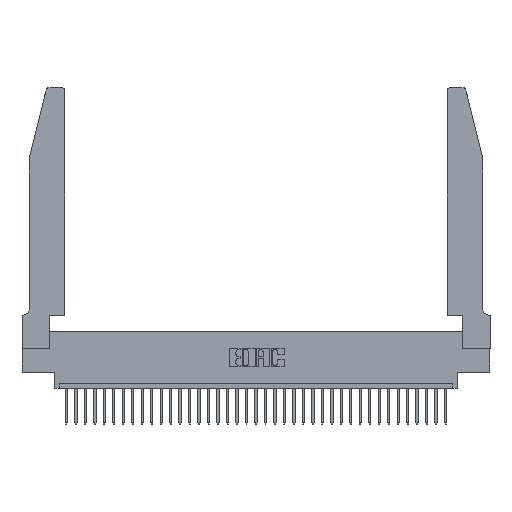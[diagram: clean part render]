
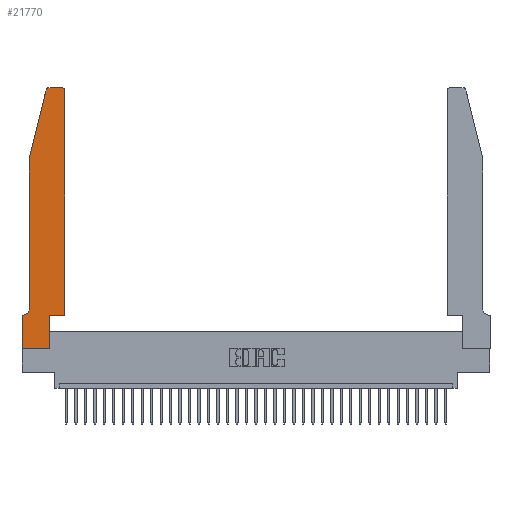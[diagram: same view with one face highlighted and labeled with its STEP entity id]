
A CAD part, top view. The second image highlights one B-rep face of the part: STEP entity #21770.
In plain terms, the highlighted planar face has unit normal (0, 0, 1).
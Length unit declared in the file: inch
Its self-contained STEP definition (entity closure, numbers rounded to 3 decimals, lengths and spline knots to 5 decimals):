
#656 = CARTESIAN_POINT ( 'NONE',  ( 0.4505, 0.35, 0.37 ) ) ;
#901 = CARTESIAN_POINT ( 'NONE',  ( 0., 0.35, 0.37 ) ) ;
#1197 = AXIS2_PLACEMENT_3D ( 'NONE', #6279, #25697, #6042 ) ;
#2085 = CARTESIAN_POINT ( 'NONE',  ( 0.0755, 0.35, 0.37 ) ) ;
#2433 = CARTESIAN_POINT ( 'NONE',  ( 0.4505, 0.35, 0.37 ) ) ;
#2552 = CARTESIAN_POINT ( 'NONE',  ( 0.4505, 0.35, 0.37 ) ) ;
#3218 = AXIS2_PLACEMENT_3D ( 'NONE', #8795, #33300, #3228 ) ;
#3228 = DIRECTION ( 'NONE',  ( 1., 0., 0. ) ) ;
#3266 = ORIENTED_EDGE ( 'NONE', *, *, #34388, .T. ) ;
#3433 = VERTEX_POINT ( 'NONE', #11619 ) ;
#3862 = DIRECTION ( 'NONE',  ( 0., -1., 0. ) ) ;
#3892 = VERTEX_POINT ( 'NONE', #28215 ) ;
#4036 = CARTESIAN_POINT ( 'NONE',  ( 0.0755, 2., 0.37 ) ) ;
#4146 = DIRECTION ( 'NONE',  ( -0.239, -0.971, 0. ) ) ;
#4921 = EDGE_CURVE ( 'NONE', #29122, #13844, #13329, .T. ) ;
#4965 = ORIENTED_EDGE ( 'NONE', *, *, #17243, .T. ) ;
#5067 = EDGE_CURVE ( 'NONE', #3433, #7374, #6825, .T. ) ;
#5284 = ORIENTED_EDGE ( 'NONE', *, *, #26502, .T. ) ;
#5329 = ORIENTED_EDGE ( 'NONE', *, *, #19090, .T. ) ;
#6042 = DIRECTION ( 'NONE',  ( 1., 0., 0. ) ) ;
#6279 = CARTESIAN_POINT ( 'NONE',  ( 0.284, 2.72, 0.37 ) ) ;
#6324 = LINE ( 'NONE', #17989, #27552 ) ;
#6640 = LINE ( 'NONE', #656, #7516 ) ;
#6825 = LINE ( 'NONE', #25083, #35454 ) ;
#7374 = VERTEX_POINT ( 'NONE', #9486 ) ;
#7516 = VECTOR ( 'NONE', #14567, 39.37008 ) ;
#7779 = AXIS2_PLACEMENT_3D ( 'NONE', #9310, #20722, #12105 ) ;
#8002 = DIRECTION ( 'NONE',  ( 1., 0., 0. ) ) ;
#8446 = DIRECTION ( 'NONE',  ( 0., 1., 0. ) ) ;
#8474 = ORIENTED_EDGE ( 'NONE', *, *, #24300, .T. ) ;
#8795 = CARTESIAN_POINT ( 'NONE',  ( 0.4205, 2.72, 0.37 ) ) ;
#9310 = CARTESIAN_POINT ( 'NONE',  ( 0.0055, 0.42, 0.37 ) ) ;
#9486 = CARTESIAN_POINT ( 'NONE',  ( 0.2865, 0.35, 0.37 ) ) ;
#9741 = EDGE_CURVE ( 'NONE', #13844, #29756, #13410, .T. ) ;
#10570 = VECTOR ( 'NONE', #32481, 39.37008 ) ;
#11619 = CARTESIAN_POINT ( 'NONE',  ( 0.2865, 0., 0.37 ) ) ;
#12105 = DIRECTION ( 'NONE',  ( -1., 0., 0. ) ) ;
#13018 = EDGE_CURVE ( 'NONE', #23200, #3433, #6324, .T. ) ;
#13329 = LINE ( 'NONE', #4036, #33725 ) ;
#13406 = EDGE_CURVE ( 'NONE', #7374, #26498, #33686, .T. ) ;
#13410 = LINE ( 'NONE', #20482, #26847 ) ;
#13844 = VERTEX_POINT ( 'NONE', #24013 ) ;
#13937 = CIRCLE ( 'NONE', #7779, 0.07 ) ;
#14264 = EDGE_LOOP ( 'NONE', ( #5284, #5329, #17696, #19869, #3266, #21389, #4965, #20018, #24490, #20926, #35298, #8474 ) ) ;
#14513 = LINE ( 'NONE', #2085, #10570 ) ;
#14567 = DIRECTION ( 'NONE',  ( 0., 1., 0. ) ) ;
#14811 = EDGE_CURVE ( 'NONE', #26498, #17972, #6640, .T. ) ;
#14813 = CARTESIAN_POINT ( 'NONE',  ( 0.0055, 0.35, 0.37 ) ) ;
#14989 = VERTEX_POINT ( 'NONE', #14813 ) ;
#16373 = CARTESIAN_POINT ( 'NONE',  ( 0.2605, 2.75, 0.37 ) ) ;
#16426 = CARTESIAN_POINT ( 'NONE',  ( 0.4505, 2.72, 0.37 ) ) ;
#16498 = LINE ( 'NONE', #16373, #30816 ) ;
#17102 = VECTOR ( 'NONE', #21934, 39.37008 ) ;
#17243 = EDGE_CURVE ( 'NONE', #26476, #23200, #24934, .T. ) ;
#17696 = ORIENTED_EDGE ( 'NONE', *, *, #4921, .T. ) ;
#17972 = VERTEX_POINT ( 'NONE', #16426 ) ;
#17989 = CARTESIAN_POINT ( 'NONE',  ( 0., 0., 0.37 ) ) ;
#19090 = EDGE_CURVE ( 'NONE', #32809, #29122, #26547, .T. ) ;
#19162 = CARTESIAN_POINT ( 'NONE',  ( 0., 0.35, 0.37 ) ) ;
#19869 = ORIENTED_EDGE ( 'NONE', *, *, #9741, .T. ) ;
#20018 = ORIENTED_EDGE ( 'NONE', *, *, #13018, .T. ) ;
#20482 = CARTESIAN_POINT ( 'NONE',  ( 0.0755, 2., 0.37 ) ) ;
#20537 = CARTESIAN_POINT ( 'NONE',  ( 0.25487, 2.72718, 0.37 ) ) ;
#20722 = DIRECTION ( 'NONE',  ( 0., 0., -1. ) ) ;
#20900 = CARTESIAN_POINT ( 'NONE',  ( 0., 0., 0.37 ) ) ;
#20926 = ORIENTED_EDGE ( 'NONE', *, *, #13406, .T. ) ;
#21389 = ORIENTED_EDGE ( 'NONE', *, *, #23517, .T. ) ;
#21770 = ADVANCED_FACE ( 'NONE', ( #25474 ), #26313, .T. ) ;
#21934 = DIRECTION ( 'NONE',  ( 0., -1., 0. ) ) ;
#23200 = VERTEX_POINT ( 'NONE', #20900 ) ;
#23295 = VECTOR ( 'NONE', #8002, 39.37008 ) ;
#23517 = EDGE_CURVE ( 'NONE', #14989, #26476, #14513, .T. ) ;
#23643 = CARTESIAN_POINT ( 'NONE',  ( 0.0755, 0.42, 0.37 ) ) ;
#23920 = DIRECTION ( 'NONE',  ( 1., 0., 0. ) ) ;
#24013 = CARTESIAN_POINT ( 'NONE',  ( 0.0755, 2., 0.37 ) ) ;
#24300 = EDGE_CURVE ( 'NONE', #17972, #3892, #26160, .T. ) ;
#24490 = ORIENTED_EDGE ( 'NONE', *, *, #5067, .T. ) ;
#24934 = LINE ( 'NONE', #32946, #17102 ) ;
#25083 = CARTESIAN_POINT ( 'NONE',  ( 0.2865, 0.35, 0.37 ) ) ;
#25474 = FACE_OUTER_BOUND ( 'NONE', #14264, .T. ) ;
#25697 = DIRECTION ( 'NONE',  ( 0., 0., 1. ) ) ;
#26160 = CIRCLE ( 'NONE', #3218, 0.03 ) ;
#26313 = PLANE ( 'NONE',  #35123 ) ;
#26476 = VERTEX_POINT ( 'NONE', #19162 ) ;
#26498 = VERTEX_POINT ( 'NONE', #2552 ) ;
#26502 = EDGE_CURVE ( 'NONE', #3892, #32809, #16498, .T. ) ;
#26547 = CIRCLE ( 'NONE', #1197, 0.03 ) ;
#26847 = VECTOR ( 'NONE', #3862, 39.37008 ) ;
#27265 = DIRECTION ( 'NONE',  ( -1., 0., 0. ) ) ;
#27552 = VECTOR ( 'NONE', #23920, 39.37008 ) ;
#28215 = CARTESIAN_POINT ( 'NONE',  ( 0.4205, 2.75, 0.37 ) ) ;
#29122 = VERTEX_POINT ( 'NONE', #20537 ) ;
#29756 = VERTEX_POINT ( 'NONE', #23643 ) ;
#29886 = CARTESIAN_POINT ( 'NONE',  ( 0.284, 2.75, 0.37 ) ) ;
#30816 = VECTOR ( 'NONE', #27265, 39.37008 ) ;
#31536 = DIRECTION ( 'NONE',  ( 0., 0., 1. ) ) ;
#32481 = DIRECTION ( 'NONE',  ( -1., 0., 0. ) ) ;
#32809 = VERTEX_POINT ( 'NONE', #29886 ) ;
#32946 = CARTESIAN_POINT ( 'NONE',  ( 0., 0., 0.37 ) ) ;
#33300 = DIRECTION ( 'NONE',  ( 0., 0., 1. ) ) ;
#33686 = LINE ( 'NONE', #2433, #23295 ) ;
#33725 = VECTOR ( 'NONE', #4146, 39.37008 ) ;
#34085 = DIRECTION ( 'NONE',  ( 1., 0., 0. ) ) ;
#34388 = EDGE_CURVE ( 'NONE', #29756, #14989, #13937, .T. ) ;
#35123 = AXIS2_PLACEMENT_3D ( 'NONE', #901, #31536, #34085 ) ;
#35298 = ORIENTED_EDGE ( 'NONE', *, *, #14811, .T. ) ;
#35454 = VECTOR ( 'NONE', #8446, 39.37008 ) ;
